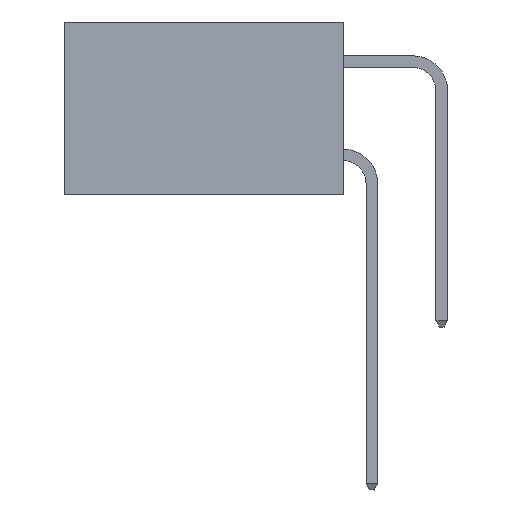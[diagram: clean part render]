
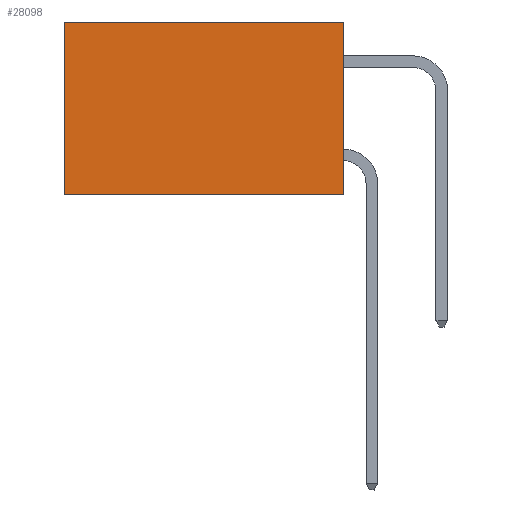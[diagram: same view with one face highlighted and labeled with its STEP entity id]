
A CAD part, left-side view. The second image highlights one B-rep face of the part: STEP entity #28098.
In plain terms, the highlighted planar face has unit normal (-1, 0, 0).
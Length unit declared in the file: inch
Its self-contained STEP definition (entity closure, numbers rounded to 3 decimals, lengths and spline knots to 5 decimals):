
#108 = VECTOR ( 'NONE', #1733, 39.37008 ) ;
#211 = ORIENTED_EDGE ( 'NONE', *, *, #23628, .F. ) ;
#1733 = DIRECTION ( 'NONE',  ( 0., 1., 0. ) ) ;
#2043 = EDGE_CURVE ( 'NONE', #19873, #6868, #5577, .T. ) ;
#2472 = VECTOR ( 'NONE', #19861, 39.37008 ) ;
#3703 = FACE_OUTER_BOUND ( 'NONE', #26133, .T. ) ;
#4179 = PLANE ( 'NONE',  #28178 ) ;
#4459 = CARTESIAN_POINT ( 'NONE',  ( 0.298, 0., -0.37 ) ) ;
#5577 = LINE ( 'NONE', #4459, #28091 ) ;
#6868 = VERTEX_POINT ( 'NONE', #11956 ) ;
#8571 = CARTESIAN_POINT ( 'NONE',  ( 0.298, 0., 0. ) ) ;
#10771 = DIRECTION ( 'NONE',  ( 1., 0., 0. ) ) ;
#11147 = ORIENTED_EDGE ( 'NONE', *, *, #14117, .T. ) ;
#11956 = CARTESIAN_POINT ( 'NONE',  ( 0.298, 0.6, -0.37 ) ) ;
#12906 = LINE ( 'NONE', #18075, #13595 ) ;
#13170 = LINE ( 'NONE', #17079, #108 ) ;
#13595 = VECTOR ( 'NONE', #20266, 39.37008 ) ;
#14117 = EDGE_CURVE ( 'NONE', #21918, #27432, #13170, .T. ) ;
#14118 = LINE ( 'NONE', #17669, #2472 ) ;
#16838 = CARTESIAN_POINT ( 'NONE',  ( 0.298, 0., 0. ) ) ;
#17079 = CARTESIAN_POINT ( 'NONE',  ( 0.298, 0., 0. ) ) ;
#17331 = CARTESIAN_POINT ( 'NONE',  ( 0.298, 0.6, 0. ) ) ;
#17669 = CARTESIAN_POINT ( 'NONE',  ( 0.298, 0.6, 0. ) ) ;
#18075 = CARTESIAN_POINT ( 'NONE',  ( 0.298, 0., 0. ) ) ;
#18892 = ORIENTED_EDGE ( 'NONE', *, *, #26181, .T. ) ;
#19861 = DIRECTION ( 'NONE',  ( 0., 0., -1. ) ) ;
#19873 = VERTEX_POINT ( 'NONE', #24787 ) ;
#20266 = DIRECTION ( 'NONE',  ( 0., 0., -1. ) ) ;
#21918 = VERTEX_POINT ( 'NONE', #16838 ) ;
#23628 = EDGE_CURVE ( 'NONE', #21918, #19873, #12906, .T. ) ;
#24170 = DIRECTION ( 'NONE',  ( 0., 1., 0. ) ) ;
#24630 = ORIENTED_EDGE ( 'NONE', *, *, #2043, .F. ) ;
#24787 = CARTESIAN_POINT ( 'NONE',  ( 0.298, 0., -0.37 ) ) ;
#25997 = DIRECTION ( 'NONE',  ( 0., 0., -1. ) ) ;
#26133 = EDGE_LOOP ( 'NONE', ( #18892, #24630, #211, #11147 ) ) ;
#26181 = EDGE_CURVE ( 'NONE', #27432, #6868, #14118, .T. ) ;
#27432 = VERTEX_POINT ( 'NONE', #17331 ) ;
#28091 = VECTOR ( 'NONE', #24170, 39.37008 ) ;
#28098 = ADVANCED_FACE ( 'NONE', ( #3703 ), #4179, .F. ) ;
#28178 = AXIS2_PLACEMENT_3D ( 'NONE', #8571, #10771, #25997 ) ;
